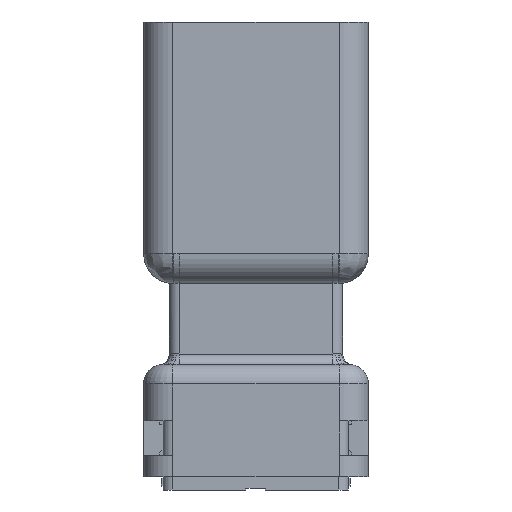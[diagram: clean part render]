
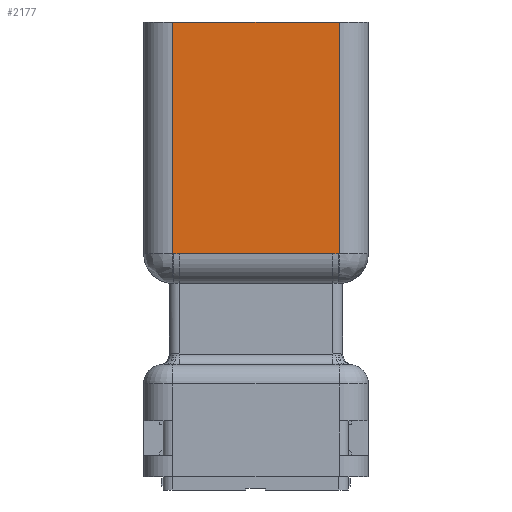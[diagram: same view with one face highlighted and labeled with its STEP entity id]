
A CAD part, front view. The second image highlights one B-rep face of the part: STEP entity #2177.
In plain terms, the highlighted planar face has unit normal (0, -1, 0).
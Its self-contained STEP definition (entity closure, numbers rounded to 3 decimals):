
#43 = CARTESIAN_POINT ( 'NONE',  ( 3.97, -3.975, 1.528 ) ) ;
#610 = VECTOR ( 'NONE', #3795, 1000. ) ;
#721 = ORIENTED_EDGE ( 'NONE', *, *, #13219, .T. ) ;
#953 = LINE ( 'NONE', #2509, #610 ) ;
#984 = DIRECTION ( 'NONE',  ( 0., 1., 0. ) ) ;
#1070 = EDGE_LOOP ( 'NONE', ( #4643, #2684, #14603, #5360, #721, #6156, #8630, #11287 ) ) ;
#1403 = EDGE_CURVE ( 'NONE', #8198, #6362, #13517, .T. ) ;
#1430 = CARTESIAN_POINT ( 'NONE',  ( 4.3, -3.975, 13.5 ) ) ;
#1484 = EDGE_CURVE ( 'NONE', #11315, #2579, #13347, .T. ) ;
#1556 = VECTOR ( 'NONE', #6057, 1000. ) ;
#2177 = ADVANCED_FACE ( 'NONE', ( #13569 ), #11926, .F. ) ;
#2509 = CARTESIAN_POINT ( 'NONE',  ( -4.3, -3.975, 1.53 ) ) ;
#2579 = VERTEX_POINT ( 'NONE', #7847 ) ;
#2684 = ORIENTED_EDGE ( 'NONE', *, *, #8918, .T. ) ;
#2780 = VECTOR ( 'NONE', #10852, 1000. ) ;
#3546 = CARTESIAN_POINT ( 'NONE',  ( -4.3, -3.975, 13.5 ) ) ;
#3612 = CARTESIAN_POINT ( 'NONE',  ( 4.063, -3.975, 1.528 ) ) ;
#3795 = DIRECTION ( 'NONE',  ( 1., 0., 0. ) ) ;
#4149 = CARTESIAN_POINT ( 'NONE',  ( -4.3, -3.975, 1.53 ) ) ;
#4643 = ORIENTED_EDGE ( 'NONE', *, *, #1403, .T. ) ;
#5360 = ORIENTED_EDGE ( 'NONE', *, *, #12992, .T. ) ;
#5487 = DIRECTION ( 'NONE',  ( 1., 0., 0. ) ) ;
#5540 = CARTESIAN_POINT ( 'NONE',  ( 4.249, -3.975, 1.53 ) ) ;
#6057 = DIRECTION ( 'NONE',  ( 1., 0., 0. ) ) ;
#6156 = ORIENTED_EDGE ( 'NONE', *, *, #1484, .T. ) ;
#6362 = VERTEX_POINT ( 'NONE', #4149 ) ;
#6412 = DIRECTION ( 'NONE',  ( 0., 0., 1. ) ) ;
#6453 = CARTESIAN_POINT ( 'NONE',  ( -4.3, -3.975, 1.53 ) ) ;
#6867 = DIRECTION ( 'NONE',  ( 0., 0., -1. ) ) ;
#6998 = B_SPLINE_CURVE_WITH_KNOTS ( 'NONE', 3,
 ( #11374, #8629, #14227, #10092 ),
 .UNSPECIFIED., .F., .F.,
 ( 4, 4 ),
 ( 0., 0. ),
 .UNSPECIFIED. ) ;
#7847 = CARTESIAN_POINT ( 'NONE',  ( 4.3, -3.975, 1.53 ) ) ;
#8040 = B_SPLINE_CURVE_WITH_KNOTS ( 'NONE', 3,
 ( #17593, #3612, #16592, #5540 ),
 .UNSPECIFIED., .F., .F.,
 ( 4, 4 ),
 ( 0., 0. ),
 .UNSPECIFIED. ) ;
#8198 = VERTEX_POINT ( 'NONE', #14349 ) ;
#8247 = LINE ( 'NONE', #9440, #8729 ) ;
#8418 = LINE ( 'NONE', #1430, #17111 ) ;
#8629 = CARTESIAN_POINT ( 'NONE',  ( -4.156, -3.975, 1.53 ) ) ;
#8630 = ORIENTED_EDGE ( 'NONE', *, *, #16001, .F. ) ;
#8729 = VECTOR ( 'NONE', #5487, 1000. ) ;
#8912 = VERTEX_POINT ( 'NONE', #17514 ) ;
#8918 = EDGE_CURVE ( 'NONE', #6362, #17644, #953, .T. ) ;
#9184 = AXIS2_PLACEMENT_3D ( 'NONE', #3546, #984, #6412 ) ;
#9440 = CARTESIAN_POINT ( 'NONE',  ( -4.3, -3.975, 1.528 ) ) ;
#10092 = CARTESIAN_POINT ( 'NONE',  ( -3.97, -3.975, 1.528 ) ) ;
#10852 = DIRECTION ( 'NONE',  ( 0., 0., -1. ) ) ;
#11287 = ORIENTED_EDGE ( 'NONE', *, *, #16655, .F. ) ;
#11315 = VERTEX_POINT ( 'NONE', #11681 ) ;
#11374 = CARTESIAN_POINT ( 'NONE',  ( -4.249, -3.975, 1.53 ) ) ;
#11681 = CARTESIAN_POINT ( 'NONE',  ( 4.249, -3.975, 1.53 ) ) ;
#11845 = CARTESIAN_POINT ( 'NONE',  ( -4.3, -3.975, 13.5 ) ) ;
#11926 = PLANE ( 'NONE',  #9184 ) ;
#12024 = VERTEX_POINT ( 'NONE', #43 ) ;
#12055 = DIRECTION ( 'NONE',  ( 1., 0., 0. ) ) ;
#12992 = EDGE_CURVE ( 'NONE', #8912, #12024, #8247, .T. ) ;
#13121 = LINE ( 'NONE', #11845, #1556 ) ;
#13219 = EDGE_CURVE ( 'NONE', #12024, #11315, #8040, .T. ) ;
#13347 = LINE ( 'NONE', #6453, #15404 ) ;
#13517 = LINE ( 'NONE', #14989, #2780 ) ;
#13569 = FACE_OUTER_BOUND ( 'NONE', #1070, .T. ) ;
#14227 = CARTESIAN_POINT ( 'NONE',  ( -4.063, -3.975, 1.528 ) ) ;
#14349 = CARTESIAN_POINT ( 'NONE',  ( -4.3, -3.975, 13.5 ) ) ;
#14603 = ORIENTED_EDGE ( 'NONE', *, *, #14779, .T. ) ;
#14779 = EDGE_CURVE ( 'NONE', #17644, #8912, #6998, .T. ) ;
#14989 = CARTESIAN_POINT ( 'NONE',  ( -4.3, -3.975, 13.5 ) ) ;
#15404 = VECTOR ( 'NONE', #12055, 1000. ) ;
#15616 = CARTESIAN_POINT ( 'NONE',  ( -4.249, -3.975, 1.53 ) ) ;
#16001 = EDGE_CURVE ( 'NONE', #17484, #2579, #8418, .T. ) ;
#16592 = CARTESIAN_POINT ( 'NONE',  ( 4.156, -3.975, 1.53 ) ) ;
#16655 = EDGE_CURVE ( 'NONE', #8198, #17484, #13121, .T. ) ;
#17111 = VECTOR ( 'NONE', #6867, 1000. ) ;
#17484 = VERTEX_POINT ( 'NONE', #18027 ) ;
#17514 = CARTESIAN_POINT ( 'NONE',  ( -3.97, -3.975, 1.528 ) ) ;
#17593 = CARTESIAN_POINT ( 'NONE',  ( 3.97, -3.975, 1.528 ) ) ;
#17644 = VERTEX_POINT ( 'NONE', #15616 ) ;
#18027 = CARTESIAN_POINT ( 'NONE',  ( 4.3, -3.975, 13.5 ) ) ;
